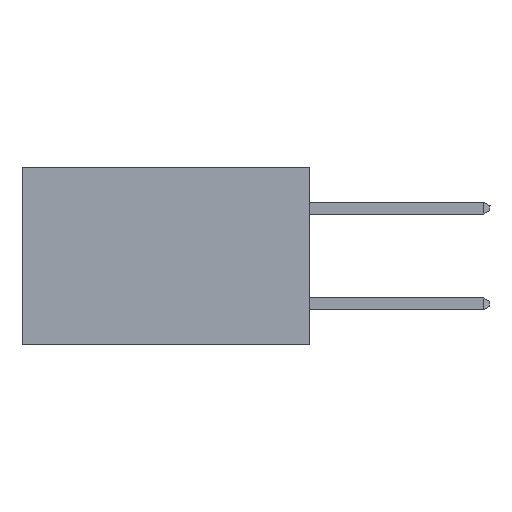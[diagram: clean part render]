
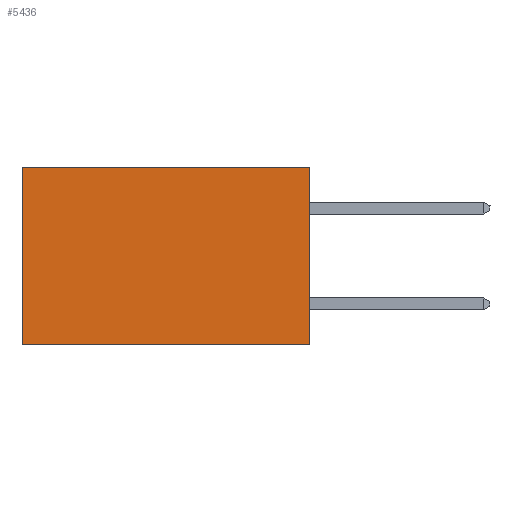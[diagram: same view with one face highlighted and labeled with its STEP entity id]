
A CAD part, left-side view. The second image highlights one B-rep face of the part: STEP entity #5436.
In plain terms, the highlighted planar face has unit normal (-1, 0, 0).
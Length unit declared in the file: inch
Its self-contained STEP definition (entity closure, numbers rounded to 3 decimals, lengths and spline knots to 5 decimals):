
#1380 = PLANE ( 'NONE',  #22976 ) ;
#1604 = VERTEX_POINT ( 'NONE', #20524 ) ;
#1771 = CARTESIAN_POINT ( 'NONE',  ( 0.2875, 0., -0.37 ) ) ;
#3269 = CARTESIAN_POINT ( 'NONE',  ( 0.2875, 0., 0. ) ) ;
#3482 = DIRECTION ( 'NONE',  ( 0., 0., -1. ) ) ;
#4435 = VECTOR ( 'NONE', #16101, 39.37008 ) ;
#4897 = VERTEX_POINT ( 'NONE', #10242 ) ;
#4980 = FACE_OUTER_BOUND ( 'NONE', #18960, .T. ) ;
#5080 = DIRECTION ( 'NONE',  ( 0., 0., -1. ) ) ;
#5436 = ADVANCED_FACE ( 'NONE', ( #4980 ), #1380, .F. ) ;
#6017 = VERTEX_POINT ( 'NONE', #25250 ) ;
#7338 = EDGE_CURVE ( 'NONE', #22157, #6017, #20132, .T. ) ;
#8548 = EDGE_CURVE ( 'NONE', #22157, #4897, #25273, .T. ) ;
#9266 = LINE ( 'NONE', #1771, #4435 ) ;
#9428 = VECTOR ( 'NONE', #13800, 39.37008 ) ;
#9732 = CARTESIAN_POINT ( 'NONE',  ( 0.2875, 0., 0. ) ) ;
#10242 = CARTESIAN_POINT ( 'NONE',  ( 0.2875, 0., -0.37 ) ) ;
#10711 = VECTOR ( 'NONE', #25916, 39.37008 ) ;
#11960 = CARTESIAN_POINT ( 'NONE',  ( 0.2875, 0.6, 0. ) ) ;
#12932 = EDGE_CURVE ( 'NONE', #6017, #1604, #16064, .T. ) ;
#13800 = DIRECTION ( 'NONE',  ( 0., 1., 0. ) ) ;
#14627 = ORIENTED_EDGE ( 'NONE', *, *, #12932, .T. ) ;
#15323 = VECTOR ( 'NONE', #5080, 39.37008 ) ;
#15730 = DIRECTION ( 'NONE',  ( 1., 0., 0. ) ) ;
#16064 = LINE ( 'NONE', #11960, #10711 ) ;
#16101 = DIRECTION ( 'NONE',  ( 0., 1., 0. ) ) ;
#16206 = ORIENTED_EDGE ( 'NONE', *, *, #7338, .T. ) ;
#17256 = CARTESIAN_POINT ( 'NONE',  ( 0.2875, 0., 0. ) ) ;
#17470 = ORIENTED_EDGE ( 'NONE', *, *, #19867, .F. ) ;
#18960 = EDGE_LOOP ( 'NONE', ( #14627, #17470, #24839, #16206 ) ) ;
#19867 = EDGE_CURVE ( 'NONE', #4897, #1604, #9266, .T. ) ;
#20132 = LINE ( 'NONE', #9732, #9428 ) ;
#20524 = CARTESIAN_POINT ( 'NONE',  ( 0.2875, 0.6, -0.37 ) ) ;
#21670 = CARTESIAN_POINT ( 'NONE',  ( 0.2875, 0., 0. ) ) ;
#22157 = VERTEX_POINT ( 'NONE', #3269 ) ;
#22976 = AXIS2_PLACEMENT_3D ( 'NONE', #21670, #15730, #3482 ) ;
#24839 = ORIENTED_EDGE ( 'NONE', *, *, #8548, .F. ) ;
#25250 = CARTESIAN_POINT ( 'NONE',  ( 0.2875, 0.6, 0. ) ) ;
#25273 = LINE ( 'NONE', #17256, #15323 ) ;
#25916 = DIRECTION ( 'NONE',  ( 0., 0., -1. ) ) ;
